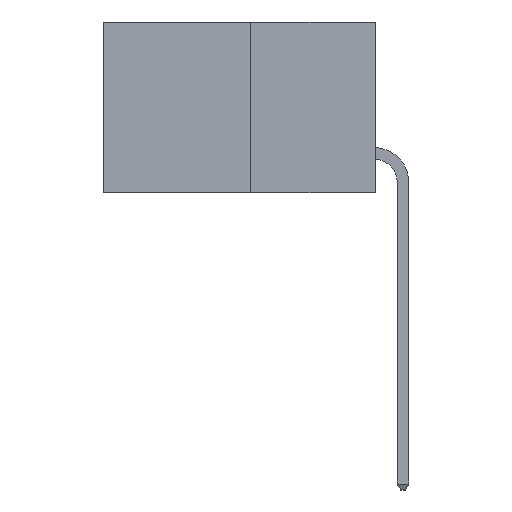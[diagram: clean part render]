
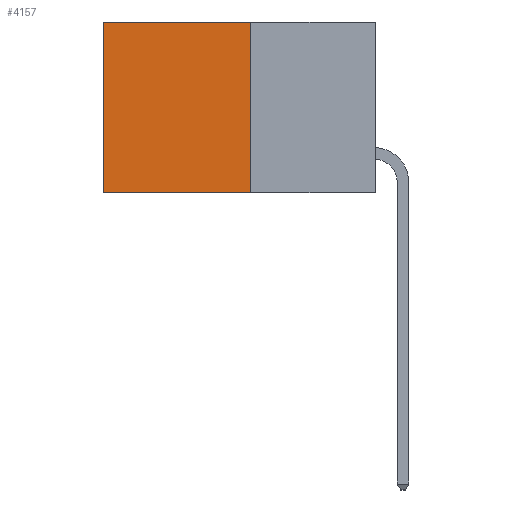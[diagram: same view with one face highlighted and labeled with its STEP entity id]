
A CAD part, left-side view. The second image highlights one B-rep face of the part: STEP entity #4157.
In plain terms, the highlighted planar face has unit normal (-1, 0, 0).
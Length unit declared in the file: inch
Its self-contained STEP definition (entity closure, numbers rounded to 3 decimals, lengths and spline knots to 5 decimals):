
#129 = EDGE_CURVE ( 'NONE', #4653, #8666, #11865, .T. ) ;
#155 = VECTOR ( 'NONE', #8697, 39.37008 ) ;
#429 = EDGE_CURVE ( 'NONE', #13646, #4653, #8980, .T. ) ;
#640 = EDGE_CURVE ( 'NONE', #13646, #4880, #3042, .T. ) ;
#1654 = CARTESIAN_POINT ( 'NONE',  ( 0.277, 0.27, 0. ) ) ;
#2054 = CARTESIAN_POINT ( 'NONE',  ( 0.277, 0.59, -0.37 ) ) ;
#3042 = LINE ( 'NONE', #12058, #5622 ) ;
#4157 = ADVANCED_FACE ( 'NONE', ( #7066 ), #12044, .F. ) ;
#4653 = VERTEX_POINT ( 'NONE', #13311 ) ;
#4833 = ORIENTED_EDGE ( 'NONE', *, *, #429, .T. ) ;
#4880 = VERTEX_POINT ( 'NONE', #10962 ) ;
#5492 = DIRECTION ( 'NONE',  ( 0., 0., -1. ) ) ;
#5622 = VECTOR ( 'NONE', #5492, 39.37008 ) ;
#5804 = VECTOR ( 'NONE', #12140, 39.37008 ) ;
#7066 = FACE_OUTER_BOUND ( 'NONE', #10296, .T. ) ;
#7159 = EDGE_CURVE ( 'NONE', #4880, #8666, #8674, .T. ) ;
#7369 = ORIENTED_EDGE ( 'NONE', *, *, #129, .T. ) ;
#8666 = VERTEX_POINT ( 'NONE', #2054 ) ;
#8674 = LINE ( 'NONE', #13656, #5804 ) ;
#8697 = DIRECTION ( 'NONE',  ( 0., 0., -1. ) ) ;
#8980 = LINE ( 'NONE', #12663, #10768 ) ;
#9705 = CARTESIAN_POINT ( 'NONE',  ( 0.277, 0.59, -0.37 ) ) ;
#10186 = ORIENTED_EDGE ( 'NONE', *, *, #7159, .F. ) ;
#10296 = EDGE_LOOP ( 'NONE', ( #7369, #10186, #12858, #4833 ) ) ;
#10768 = VECTOR ( 'NONE', #11471, 39.37008 ) ;
#10962 = CARTESIAN_POINT ( 'NONE',  ( 0.277, 0.27, -0.37 ) ) ;
#11471 = DIRECTION ( 'NONE',  ( 0., 1., 0. ) ) ;
#11865 = LINE ( 'NONE', #9705, #155 ) ;
#11907 = DIRECTION ( 'NONE',  ( 0., 0., -1. ) ) ;
#11978 = CARTESIAN_POINT ( 'NONE',  ( 0.277, 0.27, -0.37 ) ) ;
#11991 = DIRECTION ( 'NONE',  ( 1., 0., 0. ) ) ;
#12044 = PLANE ( 'NONE',  #13276 ) ;
#12058 = CARTESIAN_POINT ( 'NONE',  ( 0.277, 0.27, -0.37 ) ) ;
#12140 = DIRECTION ( 'NONE',  ( 0., 1., 0. ) ) ;
#12663 = CARTESIAN_POINT ( 'NONE',  ( 0.277, 0.27, 0. ) ) ;
#12858 = ORIENTED_EDGE ( 'NONE', *, *, #640, .F. ) ;
#13276 = AXIS2_PLACEMENT_3D ( 'NONE', #11978, #11991, #11907 ) ;
#13311 = CARTESIAN_POINT ( 'NONE',  ( 0.277, 0.59, 0. ) ) ;
#13646 = VERTEX_POINT ( 'NONE', #1654 ) ;
#13656 = CARTESIAN_POINT ( 'NONE',  ( 0.277, 0.27, -0.37 ) ) ;
